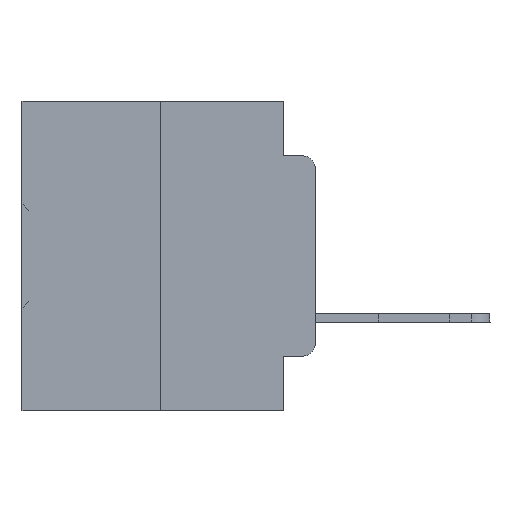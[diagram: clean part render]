
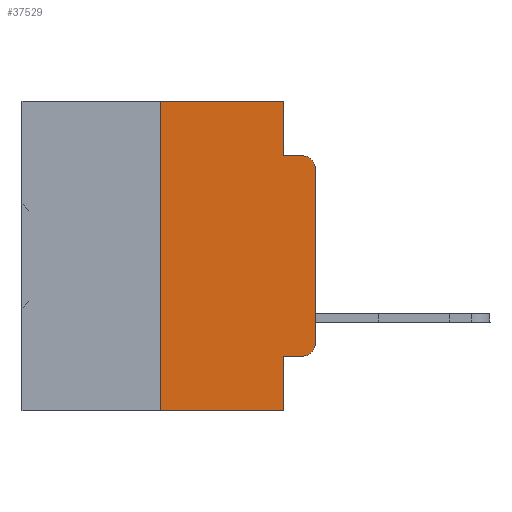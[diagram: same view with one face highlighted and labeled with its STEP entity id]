
A CAD part, left-side view. The second image highlights one B-rep face of the part: STEP entity #37529.
In plain terms, the highlighted planar face has unit normal (-1, 0, 0).
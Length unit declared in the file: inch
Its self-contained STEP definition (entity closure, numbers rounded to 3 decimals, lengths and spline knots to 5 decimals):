
#668 = CARTESIAN_POINT ( 'NONE',  ( 0., 0., -0.1085 ) ) ;
#1073 = ORIENTED_EDGE ( 'NONE', *, *, #23001, .F. ) ;
#1112 = DIRECTION ( 'NONE',  ( 0., 0., -1. ) ) ;
#1200 = VERTEX_POINT ( 'NONE', #18683 ) ;
#1634 = DIRECTION ( 'NONE',  ( -1., 0., 0. ) ) ;
#1711 = DIRECTION ( 'NONE',  ( 0., 0., -1. ) ) ;
#1895 = EDGE_CURVE ( 'NONE', #15286, #1200, #2991, .T. ) ;
#1995 = LINE ( 'NONE', #13490, #36903 ) ;
#2011 = EDGE_CURVE ( 'NONE', #17139, #25408, #25876, .T. ) ;
#2991 = LINE ( 'NONE', #28434, #7139 ) ;
#3387 = ORIENTED_EDGE ( 'NONE', *, *, #16215, .T. ) ;
#3483 = ORIENTED_EDGE ( 'NONE', *, *, #25869, .F. ) ;
#3554 = CARTESIAN_POINT ( 'NONE',  ( 0., 0.051, 0. ) ) ;
#3591 = LINE ( 'NONE', #11972, #30609 ) ;
#3642 = EDGE_CURVE ( 'NONE', #21336, #30107, #22453, .T. ) ;
#4414 = DIRECTION ( 'NONE',  ( 1., 0., 0. ) ) ;
#5168 = DIRECTION ( 'NONE',  ( 0., -1., 0. ) ) ;
#5185 = ORIENTED_EDGE ( 'NONE', *, *, #23356, .T. ) ;
#5290 = ORIENTED_EDGE ( 'NONE', *, *, #3642, .F. ) ;
#5568 = EDGE_CURVE ( 'NONE', #33229, #36281, #11103, .T. ) ;
#6391 = CARTESIAN_POINT ( 'NONE',  ( 0., 0., -0.3915 ) ) ;
#7139 = VECTOR ( 'NONE', #19696, 39.37008 ) ;
#8626 = CARTESIAN_POINT ( 'NONE',  ( 0., 0.02, -0.3915 ) ) ;
#8825 = ORIENTED_EDGE ( 'NONE', *, *, #5568, .F. ) ;
#9372 = AXIS2_PLACEMENT_3D ( 'NONE', #16591, #1634, #10712 ) ;
#9488 = CARTESIAN_POINT ( 'NONE',  ( 0., 0.473, 0. ) ) ;
#9711 = CARTESIAN_POINT ( 'NONE',  ( 0., 0.051, 0. ) ) ;
#10712 = DIRECTION ( 'NONE',  ( 0., 0., -1. ) ) ;
#11103 = LINE ( 'NONE', #3554, #20904 ) ;
#11638 = CARTESIAN_POINT ( 'NONE',  ( 0., 0.051, -0.5 ) ) ;
#11935 = DIRECTION ( 'NONE',  ( 0., 0., -1. ) ) ;
#11972 = CARTESIAN_POINT ( 'NONE',  ( 0., 0.473, -0.5 ) ) ;
#12129 = VECTOR ( 'NONE', #5168, 39.37008 ) ;
#12491 = CARTESIAN_POINT ( 'NONE',  ( 0., 0.02, -0.0885 ) ) ;
#13490 = CARTESIAN_POINT ( 'NONE',  ( 0., 0.051, -0.0885 ) ) ;
#15286 = VERTEX_POINT ( 'NONE', #27528 ) ;
#16134 = ORIENTED_EDGE ( 'NONE', *, *, #19501, .T. ) ;
#16215 = EDGE_CURVE ( 'NONE', #15286, #30107, #3591, .T. ) ;
#16268 = PLANE ( 'NONE',  #28676 ) ;
#16591 = CARTESIAN_POINT ( 'NONE',  ( 0., 0.02, -0.1085 ) ) ;
#16611 = CARTESIAN_POINT ( 'NONE',  ( 0., 0.051, -0.4115 ) ) ;
#16626 = ORIENTED_EDGE ( 'NONE', *, *, #30567, .T. ) ;
#17139 = VERTEX_POINT ( 'NONE', #34734 ) ;
#18683 = CARTESIAN_POINT ( 'NONE',  ( 0., 0.25, 0. ) ) ;
#18925 = LINE ( 'NONE', #38499, #32921 ) ;
#19100 = VERTEX_POINT ( 'NONE', #668 ) ;
#19501 = EDGE_CURVE ( 'NONE', #19100, #23526, #22075, .T. ) ;
#19696 = DIRECTION ( 'NONE',  ( 0., 0., 1. ) ) ;
#20596 = VECTOR ( 'NONE', #36433, 39.37008 ) ;
#20904 = VECTOR ( 'NONE', #1112, 39.37008 ) ;
#21336 = VERTEX_POINT ( 'NONE', #24978 ) ;
#22075 = CIRCLE ( 'NONE', #9372, 0.02 ) ;
#22453 = LINE ( 'NONE', #27442, #20596 ) ;
#22646 = LINE ( 'NONE', #9488, #34302 ) ;
#23001 = EDGE_CURVE ( 'NONE', #1200, #33229, #22646, .T. ) ;
#23200 = ORIENTED_EDGE ( 'NONE', *, *, #2011, .T. ) ;
#23356 = EDGE_CURVE ( 'NONE', #25408, #19100, #18925, .T. ) ;
#23526 = VERTEX_POINT ( 'NONE', #12491 ) ;
#23900 = AXIS2_PLACEMENT_3D ( 'NONE', #8626, #29363, #11935 ) ;
#24127 = CARTESIAN_POINT ( 'NONE',  ( 0., 0.051, -0.0885 ) ) ;
#24978 = CARTESIAN_POINT ( 'NONE',  ( 0., 0.051, -0.4115 ) ) ;
#25408 = VERTEX_POINT ( 'NONE', #6391 ) ;
#25869 = EDGE_CURVE ( 'NONE', #36281, #23526, #1995, .T. ) ;
#25876 = CIRCLE ( 'NONE', #23900, 0.02 ) ;
#27442 = CARTESIAN_POINT ( 'NONE',  ( 0., 0.051, 0. ) ) ;
#27528 = CARTESIAN_POINT ( 'NONE',  ( 0., 0.25, -0.5 ) ) ;
#27833 = FACE_OUTER_BOUND ( 'NONE', #36637, .T. ) ;
#28434 = CARTESIAN_POINT ( 'NONE',  ( 0., 0.25, 0. ) ) ;
#28676 = AXIS2_PLACEMENT_3D ( 'NONE', #34015, #4414, #1711 ) ;
#29363 = DIRECTION ( 'NONE',  ( -1., 0., 0. ) ) ;
#30107 = VERTEX_POINT ( 'NONE', #11638 ) ;
#30353 = DIRECTION ( 'NONE',  ( 0., -1., 0. ) ) ;
#30567 = EDGE_CURVE ( 'NONE', #21336, #17139, #35140, .T. ) ;
#30609 = VECTOR ( 'NONE', #36376, 39.37008 ) ;
#32609 = DIRECTION ( 'NONE',  ( 0., 0., 1. ) ) ;
#32921 = VECTOR ( 'NONE', #32609, 39.37008 ) ;
#33229 = VERTEX_POINT ( 'NONE', #9711 ) ;
#33975 = DIRECTION ( 'NONE',  ( 0., -1., 0. ) ) ;
#34015 = CARTESIAN_POINT ( 'NONE',  ( 0., 0.473, 0. ) ) ;
#34302 = VECTOR ( 'NONE', #30353, 39.37008 ) ;
#34734 = CARTESIAN_POINT ( 'NONE',  ( 0., 0.02, -0.4115 ) ) ;
#35140 = LINE ( 'NONE', #16611, #12129 ) ;
#35345 = ORIENTED_EDGE ( 'NONE', *, *, #1895, .F. ) ;
#36281 = VERTEX_POINT ( 'NONE', #24127 ) ;
#36376 = DIRECTION ( 'NONE',  ( 0., -1., 0. ) ) ;
#36433 = DIRECTION ( 'NONE',  ( 0., 0., -1. ) ) ;
#36637 = EDGE_LOOP ( 'NONE', ( #5185, #16134, #3483, #8825, #1073, #35345, #3387, #5290, #16626, #23200 ) ) ;
#36903 = VECTOR ( 'NONE', #33975, 39.37008 ) ;
#37529 = ADVANCED_FACE ( 'NONE', ( #27833 ), #16268, .F. ) ;
#38499 = CARTESIAN_POINT ( 'NONE',  ( 0., 0., 0. ) ) ;
